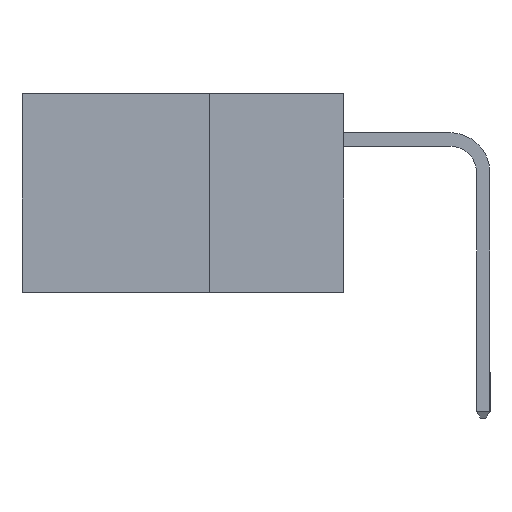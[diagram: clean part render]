
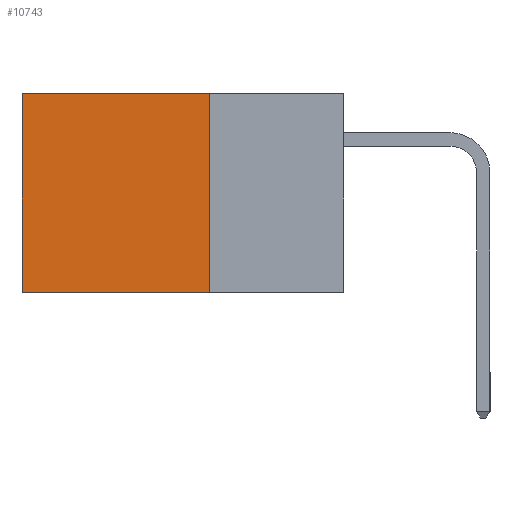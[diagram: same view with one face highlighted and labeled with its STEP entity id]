
A CAD part, left-side view. The second image highlights one B-rep face of the part: STEP entity #10743.
In plain terms, the highlighted planar face has unit normal (-1, 0, 0).
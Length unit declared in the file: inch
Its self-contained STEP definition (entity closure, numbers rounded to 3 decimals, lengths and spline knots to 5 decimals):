
#336 = VERTEX_POINT ( 'NONE', #734 ) ;
#559 = DIRECTION ( 'NONE',  ( 0., 0., -1. ) ) ;
#734 = CARTESIAN_POINT ( 'NONE',  ( 0.2615, 0.25, -0.37 ) ) ;
#1211 = AXIS2_PLACEMENT_3D ( 'NONE', #8064, #7989, #10204 ) ;
#2510 = DIRECTION ( 'NONE',  ( 0., 1., 0. ) ) ;
#3063 = VECTOR ( 'NONE', #3705, 39.37008 ) ;
#3389 = LINE ( 'NONE', #8962, #6376 ) ;
#3705 = DIRECTION ( 'NONE',  ( 0., 1., 0. ) ) ;
#4138 = CARTESIAN_POINT ( 'NONE',  ( 0.2615, 0.25, 0. ) ) ;
#4482 = FACE_OUTER_BOUND ( 'NONE', #13086, .T. ) ;
#4615 = LINE ( 'NONE', #9253, #4777 ) ;
#4644 = ORIENTED_EDGE ( 'NONE', *, *, #4682, .T. ) ;
#4682 = EDGE_CURVE ( 'NONE', #13619, #11356, #11666, .T. ) ;
#4777 = VECTOR ( 'NONE', #2510, 39.37008 ) ;
#4974 = EDGE_CURVE ( 'NONE', #8600, #13619, #7088, .T. ) ;
#5198 = VECTOR ( 'NONE', #559, 39.37008 ) ;
#6285 = EDGE_CURVE ( 'NONE', #8600, #336, #3389, .T. ) ;
#6376 = VECTOR ( 'NONE', #11365, 39.37008 ) ;
#7014 = CARTESIAN_POINT ( 'NONE',  ( 0.2615, 0.25, 0. ) ) ;
#7088 = LINE ( 'NONE', #7014, #3063 ) ;
#7989 = DIRECTION ( 'NONE',  ( 1., 0., 0. ) ) ;
#8064 = CARTESIAN_POINT ( 'NONE',  ( 0.2615, 0.25, -0.37 ) ) ;
#8323 = CARTESIAN_POINT ( 'NONE',  ( 0.2615, 0.6, -0.37 ) ) ;
#8600 = VERTEX_POINT ( 'NONE', #4138 ) ;
#8962 = CARTESIAN_POINT ( 'NONE',  ( 0.2615, 0.25, -0.37 ) ) ;
#9025 = ORIENTED_EDGE ( 'NONE', *, *, #4974, .T. ) ;
#9253 = CARTESIAN_POINT ( 'NONE',  ( 0.2615, 0.25, -0.37 ) ) ;
#9827 = ORIENTED_EDGE ( 'NONE', *, *, #12079, .F. ) ;
#9956 = ORIENTED_EDGE ( 'NONE', *, *, #6285, .F. ) ;
#10204 = DIRECTION ( 'NONE',  ( 0., 0., -1. ) ) ;
#10651 = CARTESIAN_POINT ( 'NONE',  ( 0.2615, 0.6, -0.37 ) ) ;
#10743 = ADVANCED_FACE ( 'NONE', ( #4482 ), #12258, .F. ) ;
#11049 = CARTESIAN_POINT ( 'NONE',  ( 0.2615, 0.6, 0. ) ) ;
#11356 = VERTEX_POINT ( 'NONE', #8323 ) ;
#11365 = DIRECTION ( 'NONE',  ( 0., 0., -1. ) ) ;
#11666 = LINE ( 'NONE', #10651, #5198 ) ;
#12079 = EDGE_CURVE ( 'NONE', #336, #11356, #4615, .T. ) ;
#12258 = PLANE ( 'NONE',  #1211 ) ;
#13086 = EDGE_LOOP ( 'NONE', ( #4644, #9827, #9956, #9025 ) ) ;
#13619 = VERTEX_POINT ( 'NONE', #11049 ) ;
